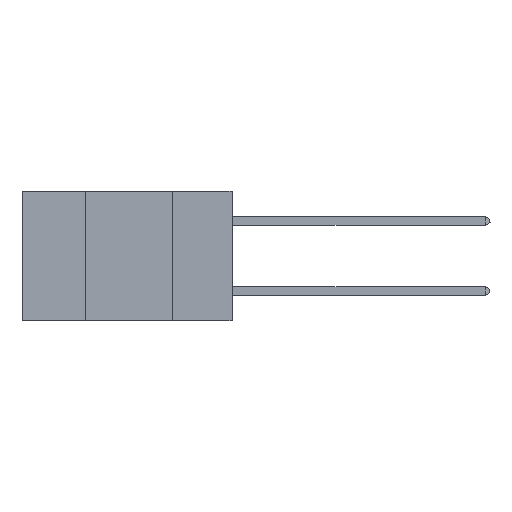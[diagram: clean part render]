
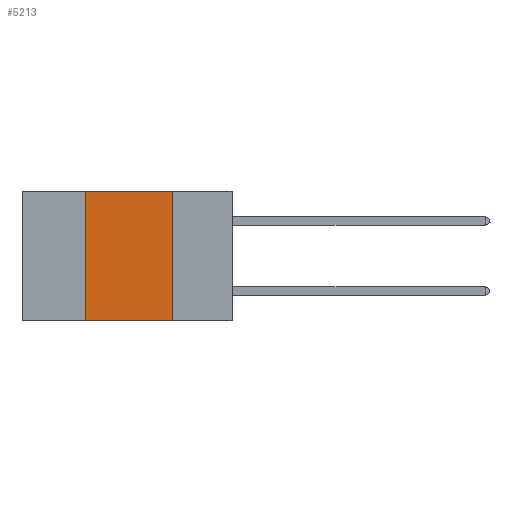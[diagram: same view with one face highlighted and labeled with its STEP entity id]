
A CAD part, left-side view. The second image highlights one B-rep face of the part: STEP entity #5213.
In plain terms, the highlighted planar face has unit normal (-1, 0, 0).
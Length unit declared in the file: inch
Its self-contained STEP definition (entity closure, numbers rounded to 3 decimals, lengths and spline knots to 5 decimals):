
#214 = DIRECTION ( 'NONE',  ( 0., -1., 0. ) ) ;
#496 = VECTOR ( 'NONE', #6451, 39.37008 ) ;
#1382 = CARTESIAN_POINT ( 'NONE',  ( 0., 0.42, -0.37 ) ) ;
#1453 = LINE ( 'NONE', #8055, #1819 ) ;
#1819 = VECTOR ( 'NONE', #6066, 39.37008 ) ;
#1950 = VECTOR ( 'NONE', #214, 39.37008 ) ;
#1955 = CARTESIAN_POINT ( 'NONE',  ( 0., 0.6, 0. ) ) ;
#2437 = CARTESIAN_POINT ( 'NONE',  ( 0., 0.17, 0. ) ) ;
#2690 = VECTOR ( 'NONE', #4964, 39.37008 ) ;
#3138 = CARTESIAN_POINT ( 'NONE',  ( 0., 0.6, 0. ) ) ;
#3240 = ORIENTED_EDGE ( 'NONE', *, *, #4710, .F. ) ;
#3803 = EDGE_CURVE ( 'NONE', #11287, #9999, #9117, .T. ) ;
#3827 = CARTESIAN_POINT ( 'NONE',  ( 0., 0.42, 0. ) ) ;
#4055 = DIRECTION ( 'NONE',  ( 1., 0., 0. ) ) ;
#4710 = EDGE_CURVE ( 'NONE', #11287, #11236, #9318, .T. ) ;
#4964 = DIRECTION ( 'NONE',  ( 0., 0., 1. ) ) ;
#5213 = ADVANCED_FACE ( 'NONE', ( #8692 ), #9598, .F. ) ;
#5890 = CARTESIAN_POINT ( 'NONE',  ( 0., 0.42, 0. ) ) ;
#6066 = DIRECTION ( 'NONE',  ( 0., 0., -1. ) ) ;
#6166 = CARTESIAN_POINT ( 'NONE',  ( 0., 0.17, -0.37 ) ) ;
#6451 = DIRECTION ( 'NONE',  ( 0., -1., 0. ) ) ;
#6543 = EDGE_LOOP ( 'NONE', ( #8740, #10004, #3240, #10801 ) ) ;
#7895 = AXIS2_PLACEMENT_3D ( 'NONE', #3138, #4055, #10368 ) ;
#8055 = CARTESIAN_POINT ( 'NONE',  ( 0., 0.17, 0. ) ) ;
#8692 = FACE_OUTER_BOUND ( 'NONE', #6543, .T. ) ;
#8740 = ORIENTED_EDGE ( 'NONE', *, *, #11390, .F. ) ;
#9117 = LINE ( 'NONE', #9303, #1950 ) ;
#9303 = CARTESIAN_POINT ( 'NONE',  ( 0., 0.6, -0.37 ) ) ;
#9318 = LINE ( 'NONE', #3827, #2690 ) ;
#9598 = PLANE ( 'NONE',  #7895 ) ;
#9999 = VERTEX_POINT ( 'NONE', #6166 ) ;
#10004 = ORIENTED_EDGE ( 'NONE', *, *, #10127, .F. ) ;
#10127 = EDGE_CURVE ( 'NONE', #11236, #10569, #11092, .T. ) ;
#10368 = DIRECTION ( 'NONE',  ( 0., 0., -1. ) ) ;
#10569 = VERTEX_POINT ( 'NONE', #2437 ) ;
#10801 = ORIENTED_EDGE ( 'NONE', *, *, #3803, .T. ) ;
#11092 = LINE ( 'NONE', #1955, #496 ) ;
#11236 = VERTEX_POINT ( 'NONE', #5890 ) ;
#11287 = VERTEX_POINT ( 'NONE', #1382 ) ;
#11390 = EDGE_CURVE ( 'NONE', #10569, #9999, #1453, .T. ) ;
